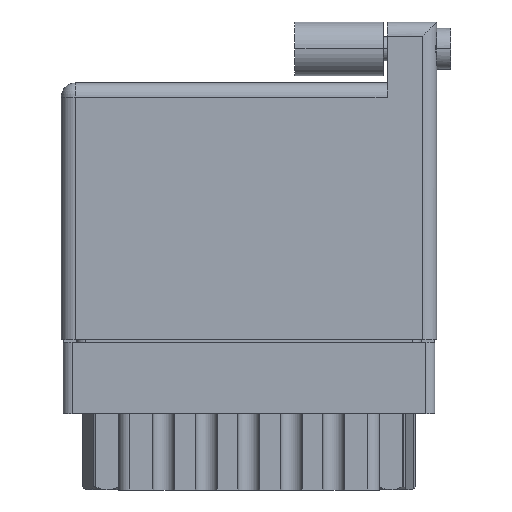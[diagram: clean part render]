
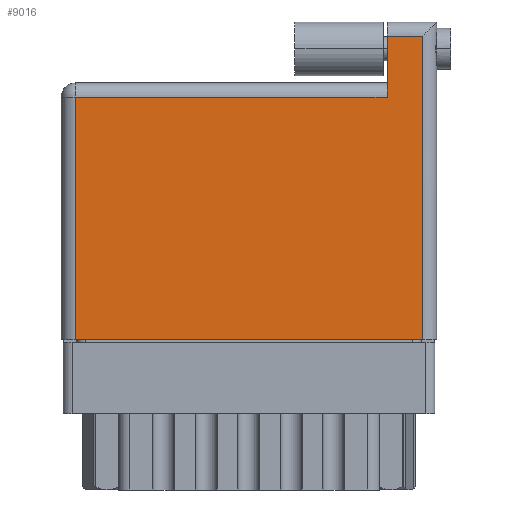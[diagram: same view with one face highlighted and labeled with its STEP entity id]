
A CAD part, front view. The second image highlights one B-rep face of the part: STEP entity #9016.
In plain terms, the highlighted face is planar.
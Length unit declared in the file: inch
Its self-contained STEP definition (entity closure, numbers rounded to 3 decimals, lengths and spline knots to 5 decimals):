
#1569 = EDGE_CURVE ( 'NONE', #27637, #14206, #1877, .T. ) ;
#1870 = CARTESIAN_POINT ( 'NONE',  ( 1.275, 0., 0. ) ) ;
#1877 = LINE ( 'NONE', #8227, #8899 ) ;
#1970 = VECTOR ( 'NONE', #20390, 39.37008 ) ;
#2694 = CARTESIAN_POINT ( 'NONE',  ( 1.275, 1.07, 0. ) ) ;
#3182 = CARTESIAN_POINT ( 'NONE',  ( 0., 0., 0. ) ) ;
#4457 = EDGE_CURVE ( 'NONE', #20665, #28082, #12773, .T. ) ;
#4555 = LINE ( 'NONE', #5247, #25872 ) ;
#4589 = CARTESIAN_POINT ( 'NONE',  ( 0.05, 0.856, 0. ) ) ;
#5013 = FACE_OUTER_BOUND ( 'NONE', #20650, .T. ) ;
#5247 = CARTESIAN_POINT ( 'NONE',  ( 0., 0.856, 0. ) ) ;
#6634 = PLANE ( 'NONE',  #30554 ) ;
#7294 = EDGE_CURVE ( 'NONE', #14206, #26867, #21664, .T. ) ;
#7823 = DIRECTION ( 'NONE',  ( -1., 0., 0. ) ) ;
#8227 = CARTESIAN_POINT ( 'NONE',  ( 0., 1.07, 0. ) ) ;
#8478 = CARTESIAN_POINT ( 'NONE',  ( 1.15, 0.856, 0. ) ) ;
#8879 = LINE ( 'NONE', #3182, #29308 ) ;
#8899 = VECTOR ( 'NONE', #14058, 39.37008 ) ;
#8961 = EDGE_CURVE ( 'NONE', #32548, #27637, #29835, .T. ) ;
#9016 = ADVANCED_FACE ( 'NONE', ( #5013 ), #6634, .F. ) ;
#11483 = DIRECTION ( 'NONE',  ( 0., -1., 0. ) ) ;
#12773 = LINE ( 'NONE', #19741, #14526 ) ;
#13230 = CARTESIAN_POINT ( 'NONE',  ( 1.15, 1.07, 0. ) ) ;
#13365 = ORIENTED_EDGE ( 'NONE', *, *, #4457, .T. ) ;
#14058 = DIRECTION ( 'NONE',  ( -1., 0., 0. ) ) ;
#14206 = VERTEX_POINT ( 'NONE', #13230 ) ;
#14526 = VECTOR ( 'NONE', #11483, 39.37008 ) ;
#15189 = EDGE_CURVE ( 'NONE', #28082, #32548, #8879, .T. ) ;
#15575 = DIRECTION ( 'NONE',  ( 1., 0., 0. ) ) ;
#19741 = CARTESIAN_POINT ( 'NONE',  ( 0.05, 0., 0. ) ) ;
#20060 = ORIENTED_EDGE ( 'NONE', *, *, #15189, .T. ) ;
#20390 = DIRECTION ( 'NONE',  ( 0., 1., 0. ) ) ;
#20650 = EDGE_LOOP ( 'NONE', ( #20060, #30280, #28863, #35138, #25092, #13365 ) ) ;
#20665 = VERTEX_POINT ( 'NONE', #4589 ) ;
#21664 = LINE ( 'NONE', #35994, #31719 ) ;
#22695 = EDGE_CURVE ( 'NONE', #26867, #20665, #4555, .T. ) ;
#24683 = CARTESIAN_POINT ( 'NONE',  ( 0.05, 0., 0. ) ) ;
#25092 = ORIENTED_EDGE ( 'NONE', *, *, #22695, .T. ) ;
#25872 = VECTOR ( 'NONE', #7823, 39.37008 ) ;
#26867 = VERTEX_POINT ( 'NONE', #8478 ) ;
#27365 = DIRECTION ( 'NONE',  ( 0., -1., 0. ) ) ;
#27637 = VERTEX_POINT ( 'NONE', #2694 ) ;
#28082 = VERTEX_POINT ( 'NONE', #24683 ) ;
#28503 = CARTESIAN_POINT ( 'NONE',  ( 1.275, 1.12, 0. ) ) ;
#28863 = ORIENTED_EDGE ( 'NONE', *, *, #1569, .T. ) ;
#28867 = CARTESIAN_POINT ( 'NONE',  ( 0., 0.906, 0. ) ) ;
#29308 = VECTOR ( 'NONE', #15575, 39.37008 ) ;
#29835 = LINE ( 'NONE', #28503, #1970 ) ;
#30280 = ORIENTED_EDGE ( 'NONE', *, *, #8961, .T. ) ;
#30554 = AXIS2_PLACEMENT_3D ( 'NONE', #28867, #31345, #31473 ) ;
#31345 = DIRECTION ( 'NONE',  ( 0., 0., -1. ) ) ;
#31473 = DIRECTION ( 'NONE',  ( -1., 0., 0. ) ) ;
#31719 = VECTOR ( 'NONE', #27365, 39.37008 ) ;
#32548 = VERTEX_POINT ( 'NONE', #1870 ) ;
#35138 = ORIENTED_EDGE ( 'NONE', *, *, #7294, .T. ) ;
#35994 = CARTESIAN_POINT ( 'NONE',  ( 1.15, 1.12, 0. ) ) ;
